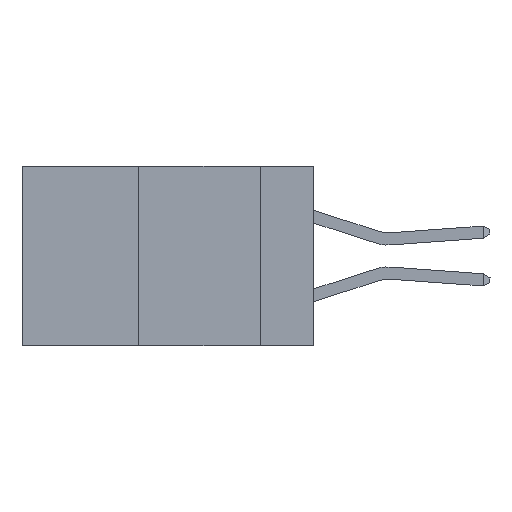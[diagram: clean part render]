
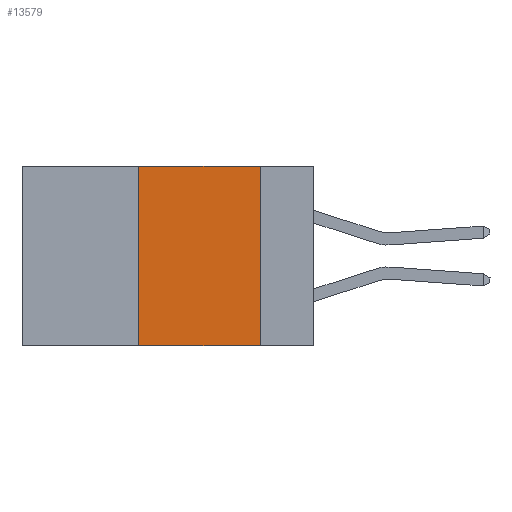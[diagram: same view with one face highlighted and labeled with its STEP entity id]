
A CAD part, left-side view. The second image highlights one B-rep face of the part: STEP entity #13579.
In plain terms, the highlighted planar face has unit normal (-1, 0, 0).
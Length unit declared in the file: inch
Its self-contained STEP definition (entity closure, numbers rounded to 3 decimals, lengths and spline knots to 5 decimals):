
#222 = FACE_OUTER_BOUND ( 'NONE', #13303, .T. ) ;
#389 = LINE ( 'NONE', #3753, #18543 ) ;
#1258 = DIRECTION ( 'NONE',  ( 1., 0., 0. ) ) ;
#2736 = EDGE_CURVE ( 'NONE', #17254, #11881, #16189, .T. ) ;
#2808 = CARTESIAN_POINT ( 'NONE',  ( 0., 0.6, 0. ) ) ;
#2946 = DIRECTION ( 'NONE',  ( 0., -1., 0. ) ) ;
#3448 = CARTESIAN_POINT ( 'NONE',  ( 0., 0.11, -0.37 ) ) ;
#3572 = EDGE_CURVE ( 'NONE', #14967, #17254, #18709, .T. ) ;
#3753 = CARTESIAN_POINT ( 'NONE',  ( 0., 0.36, 0. ) ) ;
#4800 = DIRECTION ( 'NONE',  ( 0., -1., 0. ) ) ;
#5583 = ORIENTED_EDGE ( 'NONE', *, *, #3572, .F. ) ;
#5909 = EDGE_CURVE ( 'NONE', #13199, #11881, #8726, .T. ) ;
#7362 = ORIENTED_EDGE ( 'NONE', *, *, #9905, .F. ) ;
#8726 = LINE ( 'NONE', #9646, #12734 ) ;
#9351 = AXIS2_PLACEMENT_3D ( 'NONE', #18941, #1258, #17006 ) ;
#9646 = CARTESIAN_POINT ( 'NONE',  ( 0., 0.6, -0.37 ) ) ;
#9905 = EDGE_CURVE ( 'NONE', #13199, #14967, #389, .T. ) ;
#10658 = CARTESIAN_POINT ( 'NONE',  ( 0., 0.11, 0. ) ) ;
#10848 = PLANE ( 'NONE',  #9351 ) ;
#11616 = VECTOR ( 'NONE', #18963, 39.37008 ) ;
#11881 = VERTEX_POINT ( 'NONE', #3448 ) ;
#12734 = VECTOR ( 'NONE', #4800, 39.37008 ) ;
#13199 = VERTEX_POINT ( 'NONE', #15676 ) ;
#13303 = EDGE_LOOP ( 'NONE', ( #19713, #5583, #7362, #16977 ) ) ;
#13579 = ADVANCED_FACE ( 'NONE', ( #222 ), #10848, .F. ) ;
#14967 = VERTEX_POINT ( 'NONE', #15179 ) ;
#15179 = CARTESIAN_POINT ( 'NONE',  ( 0., 0.36, 0. ) ) ;
#15649 = VECTOR ( 'NONE', #2946, 39.37008 ) ;
#15676 = CARTESIAN_POINT ( 'NONE',  ( 0., 0.36, -0.37 ) ) ;
#16189 = LINE ( 'NONE', #18813, #11616 ) ;
#16519 = DIRECTION ( 'NONE',  ( 0., 0., 1. ) ) ;
#16977 = ORIENTED_EDGE ( 'NONE', *, *, #5909, .T. ) ;
#17006 = DIRECTION ( 'NONE',  ( 0., 0., -1. ) ) ;
#17254 = VERTEX_POINT ( 'NONE', #10658 ) ;
#18543 = VECTOR ( 'NONE', #16519, 39.37008 ) ;
#18709 = LINE ( 'NONE', #2808, #15649 ) ;
#18813 = CARTESIAN_POINT ( 'NONE',  ( 0., 0.11, 0. ) ) ;
#18941 = CARTESIAN_POINT ( 'NONE',  ( 0., 0.6, 0. ) ) ;
#18963 = DIRECTION ( 'NONE',  ( 0., 0., -1. ) ) ;
#19713 = ORIENTED_EDGE ( 'NONE', *, *, #2736, .F. ) ;
